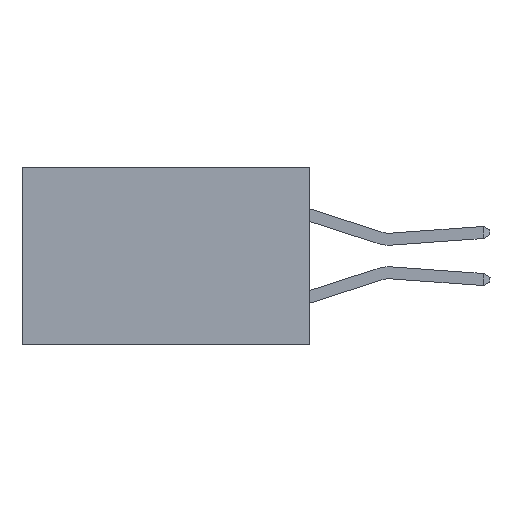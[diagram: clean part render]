
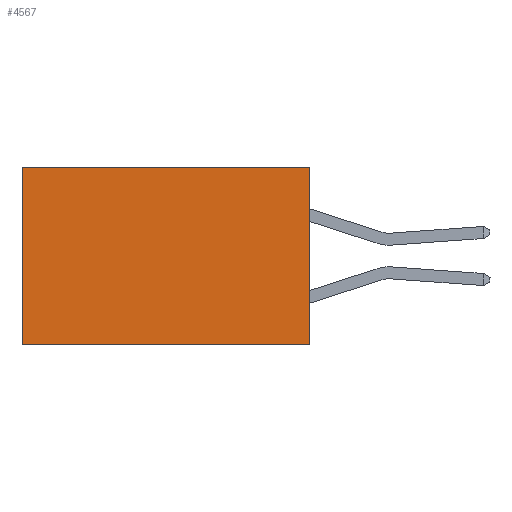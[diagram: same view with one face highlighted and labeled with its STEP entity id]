
A CAD part, left-side view. The second image highlights one B-rep face of the part: STEP entity #4567.
In plain terms, the highlighted planar face has unit normal (-1, 0, 0).
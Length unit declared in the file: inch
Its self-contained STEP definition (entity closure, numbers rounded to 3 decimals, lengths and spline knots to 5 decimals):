
#4 = DIRECTION ( 'NONE',  ( 0., 1., 0. ) ) ;
#83 = EDGE_CURVE ( 'NONE', #216, #8067, #8001, .T. ) ;
#182 = DIRECTION ( 'NONE',  ( 0., 0., -1. ) ) ;
#216 = VERTEX_POINT ( 'NONE', #3820 ) ;
#505 = VECTOR ( 'NONE', #182, 39.37008 ) ;
#652 = VERTEX_POINT ( 'NONE', #6468 ) ;
#766 = PLANE ( 'NONE',  #3133 ) ;
#979 = VECTOR ( 'NONE', #7632, 39.37008 ) ;
#1707 = EDGE_CURVE ( 'NONE', #652, #8067, #6127, .T. ) ;
#1733 = DIRECTION ( 'NONE',  ( 0., 1., 0. ) ) ;
#1808 = LINE ( 'NONE', #7216, #6603 ) ;
#2166 = FACE_OUTER_BOUND ( 'NONE', #7365, .T. ) ;
#2200 = DIRECTION ( 'NONE',  ( 0., 0., -1. ) ) ;
#2474 = VERTEX_POINT ( 'NONE', #7850 ) ;
#3133 = AXIS2_PLACEMENT_3D ( 'NONE', #6412, #7214, #2200 ) ;
#3143 = EDGE_CURVE ( 'NONE', #2474, #216, #1808, .T. ) ;
#3532 = CARTESIAN_POINT ( 'NONE',  ( 0.298, 0., 0. ) ) ;
#3820 = CARTESIAN_POINT ( 'NONE',  ( 0.298, 0.6, 0. ) ) ;
#4101 = EDGE_CURVE ( 'NONE', #2474, #652, #9652, .T. ) ;
#4567 = ADVANCED_FACE ( 'NONE', ( #2166 ), #766, .F. ) ;
#5107 = VECTOR ( 'NONE', #4, 39.37008 ) ;
#5822 = CARTESIAN_POINT ( 'NONE',  ( 0.298, 0., -0.37 ) ) ;
#6127 = LINE ( 'NONE', #5822, #5107 ) ;
#6412 = CARTESIAN_POINT ( 'NONE',  ( 0.298, 0., 0. ) ) ;
#6468 = CARTESIAN_POINT ( 'NONE',  ( 0.298, 0., -0.37 ) ) ;
#6603 = VECTOR ( 'NONE', #1733, 39.37008 ) ;
#6625 = ORIENTED_EDGE ( 'NONE', *, *, #4101, .F. ) ;
#6811 = ORIENTED_EDGE ( 'NONE', *, *, #3143, .T. ) ;
#7214 = DIRECTION ( 'NONE',  ( 1., 0., 0. ) ) ;
#7216 = CARTESIAN_POINT ( 'NONE',  ( 0.298, 0., 0. ) ) ;
#7365 = EDGE_LOOP ( 'NONE', ( #9586, #7703, #6625, #6811 ) ) ;
#7632 = DIRECTION ( 'NONE',  ( 0., 0., -1. ) ) ;
#7703 = ORIENTED_EDGE ( 'NONE', *, *, #1707, .F. ) ;
#7714 = CARTESIAN_POINT ( 'NONE',  ( 0.298, 0.6, -0.37 ) ) ;
#7850 = CARTESIAN_POINT ( 'NONE',  ( 0.298, 0., 0. ) ) ;
#8001 = LINE ( 'NONE', #9205, #979 ) ;
#8067 = VERTEX_POINT ( 'NONE', #7714 ) ;
#9205 = CARTESIAN_POINT ( 'NONE',  ( 0.298, 0.6, 0. ) ) ;
#9586 = ORIENTED_EDGE ( 'NONE', *, *, #83, .T. ) ;
#9652 = LINE ( 'NONE', #3532, #505 ) ;
